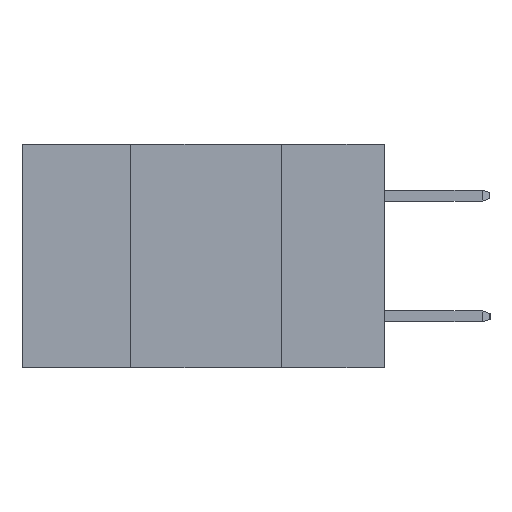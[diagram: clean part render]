
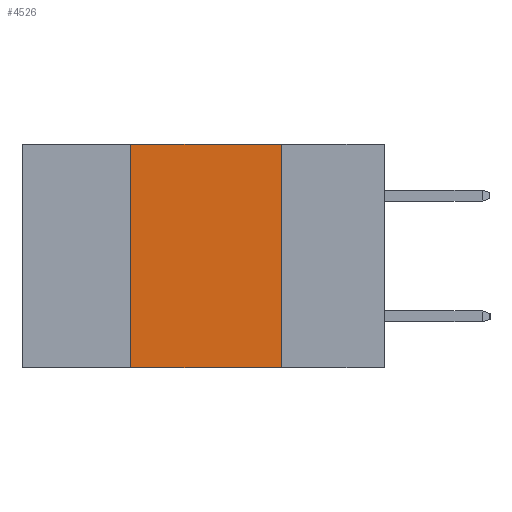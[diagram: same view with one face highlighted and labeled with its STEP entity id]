
A CAD part, left-side view. The second image highlights one B-rep face of the part: STEP entity #4526.
In plain terms, the highlighted planar face has unit normal (-1, 0, 0).
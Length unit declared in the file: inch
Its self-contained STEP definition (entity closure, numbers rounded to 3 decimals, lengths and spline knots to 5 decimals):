
#360 = AXIS2_PLACEMENT_3D ( 'NONE', #9345, #7643, #7525 ) ;
#606 = CARTESIAN_POINT ( 'NONE',  ( 0., 0.42, 0. ) ) ;
#1683 = LINE ( 'NONE', #9890, #10765 ) ;
#2078 = CARTESIAN_POINT ( 'NONE',  ( 0., 0.17, 0. ) ) ;
#2731 = VECTOR ( 'NONE', #7810, 39.37008 ) ;
#2917 = VECTOR ( 'NONE', #7794, 39.37008 ) ;
#3966 = LINE ( 'NONE', #9479, #8434 ) ;
#4214 = CARTESIAN_POINT ( 'NONE',  ( 0., 0.6, -0.37 ) ) ;
#4245 = FACE_OUTER_BOUND ( 'NONE', #9727, .T. ) ;
#4526 = ADVANCED_FACE ( 'NONE', ( #4245 ), #7775, .F. ) ;
#4840 = EDGE_CURVE ( 'NONE', #7773, #7448, #1683, .T. ) ;
#4952 = EDGE_CURVE ( 'NONE', #10942, #7773, #3966, .T. ) ;
#5154 = EDGE_CURVE ( 'NONE', #7448, #8433, #9760, .T. ) ;
#5205 = ORIENTED_EDGE ( 'NONE', *, *, #4952, .F. ) ;
#5487 = ORIENTED_EDGE ( 'NONE', *, *, #4840, .F. ) ;
#5977 = LINE ( 'NONE', #4214, #2917 ) ;
#7288 = ORIENTED_EDGE ( 'NONE', *, *, #9402, .T. ) ;
#7448 = VERTEX_POINT ( 'NONE', #2078 ) ;
#7525 = DIRECTION ( 'NONE',  ( 0., 0., -1. ) ) ;
#7643 = DIRECTION ( 'NONE',  ( 1., 0., 0. ) ) ;
#7773 = VERTEX_POINT ( 'NONE', #606 ) ;
#7775 = PLANE ( 'NONE',  #360 ) ;
#7794 = DIRECTION ( 'NONE',  ( 0., -1., 0. ) ) ;
#7810 = DIRECTION ( 'NONE',  ( 0., 0., -1. ) ) ;
#7849 = CARTESIAN_POINT ( 'NONE',  ( 0., 0.42, -0.37 ) ) ;
#7999 = CARTESIAN_POINT ( 'NONE',  ( 0., 0.17, -0.37 ) ) ;
#8433 = VERTEX_POINT ( 'NONE', #8553 ) ;
#8434 = VECTOR ( 'NONE', #9642, 39.37008 ) ;
#8553 = CARTESIAN_POINT ( 'NONE',  ( 0., 0.17, -0.37 ) ) ;
#9345 = CARTESIAN_POINT ( 'NONE',  ( 0., 0.6, 0. ) ) ;
#9402 = EDGE_CURVE ( 'NONE', #10942, #8433, #5977, .T. ) ;
#9479 = CARTESIAN_POINT ( 'NONE',  ( 0., 0.42, -0.37 ) ) ;
#9642 = DIRECTION ( 'NONE',  ( 0., 0., 1. ) ) ;
#9727 = EDGE_LOOP ( 'NONE', ( #10929, #5487, #5205, #7288 ) ) ;
#9760 = LINE ( 'NONE', #7999, #2731 ) ;
#9824 = DIRECTION ( 'NONE',  ( 0., -1., 0. ) ) ;
#9890 = CARTESIAN_POINT ( 'NONE',  ( 0., 0.6, 0. ) ) ;
#10765 = VECTOR ( 'NONE', #9824, 39.37008 ) ;
#10929 = ORIENTED_EDGE ( 'NONE', *, *, #5154, .F. ) ;
#10942 = VERTEX_POINT ( 'NONE', #7849 ) ;
